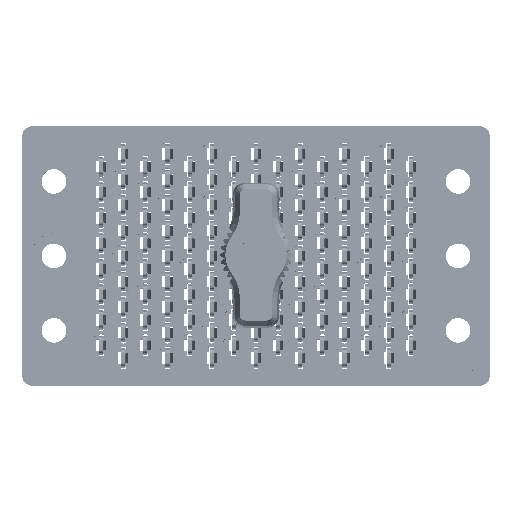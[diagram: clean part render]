
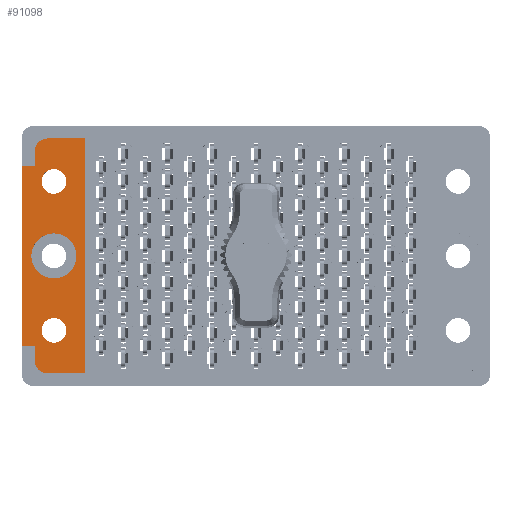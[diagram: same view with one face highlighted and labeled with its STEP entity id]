
A CAD part, top view. The second image highlights one B-rep face of the part: STEP entity #91098.
In plain terms, the highlighted planar face has unit normal (0, 0, 1).
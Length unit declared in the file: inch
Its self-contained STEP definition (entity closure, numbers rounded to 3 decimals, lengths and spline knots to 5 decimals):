
#520 = EDGE_CURVE ( 'NONE', #76508, #47796, #1951, .T. ) ;
#1688 = CARTESIAN_POINT ( 'NONE',  ( -1.3, 0.5285, -0.117 ) ) ;
#1951 = LINE ( 'NONE', #77015, #81030 ) ;
#3265 = VERTEX_POINT ( 'NONE', #38619 ) ;
#3399 = CARTESIAN_POINT ( 'NONE',  ( -1.225, -0.615, -0.117 ) ) ;
#4760 = VECTOR ( 'NONE', #86112, 39.37008 ) ;
#5587 = DIRECTION ( 'NONE',  ( 1., 0., 0. ) ) ;
#7339 = CARTESIAN_POINT ( 'NONE',  ( -1.3, -0.615, -0.117 ) ) ;
#7540 = DIRECTION ( 'NONE',  ( -1., 0., 0. ) ) ;
#8501 = VERTEX_POINT ( 'NONE', #13910 ) ;
#8773 = EDGE_LOOP ( 'NONE', ( #49621, #72339 ) ) ;
#10716 = DIRECTION ( 'NONE',  ( 0., 0., 1. ) ) ;
#10899 = VERTEX_POINT ( 'NONE', #83333 ) ;
#11388 = DIRECTION ( 'NONE',  ( -1., 0., 0. ) ) ;
#11591 = EDGE_LOOP ( 'NONE', ( #106230, #72135 ) ) ;
#11760 = CARTESIAN_POINT ( 'NONE',  ( 0., 0.69, -0.117 ) ) ;
#11812 = VERTEX_POINT ( 'NONE', #95992 ) ;
#11951 = AXIS2_PLACEMENT_3D ( 'NONE', #38416, #14511, #63714 ) ;
#12415 = VERTEX_POINT ( 'NONE', #104244 ) ;
#12873 = VECTOR ( 'NONE', #105240, 39.37008 ) ;
#13069 = VERTEX_POINT ( 'NONE', #104713 ) ;
#13159 = VERTEX_POINT ( 'NONE', #7339 ) ;
#13910 = CARTESIAN_POINT ( 'NONE',  ( -1.115, 0.4375, -0.117 ) ) ;
#14511 = DIRECTION ( 'NONE',  ( 0., 0., 1. ) ) ;
#15698 = EDGE_CURVE ( 'NONE', #92973, #13069, #87739, .T. ) ;
#16924 = ORIENTED_EDGE ( 'NONE', *, *, #95785, .F. ) ;
#18304 = CIRCLE ( 'NONE', #53966, 0.1325 ) ;
#19270 = DIRECTION ( 'NONE',  ( 1., 0., 0. ) ) ;
#19272 = VECTOR ( 'NONE', #11388, 39.37008 ) ;
#19824 = DIRECTION ( 'NONE',  ( 1., 0., 0. ) ) ;
#19916 = FACE_OUTER_BOUND ( 'NONE', #60039, .T. ) ;
#21503 = ORIENTED_EDGE ( 'NONE', *, *, #50253, .T. ) ;
#21797 = VECTOR ( 'NONE', #71695, 39.37008 ) ;
#23635 = VERTEX_POINT ( 'NONE', #99244 ) ;
#23939 = CARTESIAN_POINT ( 'NONE',  ( -1.1875, -0.4375, -0.117 ) ) ;
#25273 = CARTESIAN_POINT ( 'NONE',  ( -1.26, 0.4375, -0.117 ) ) ;
#25336 = CIRCLE ( 'NONE', #72928, 0.1325 ) ;
#26126 = ORIENTED_EDGE ( 'NONE', *, *, #47412, .T. ) ;
#26280 = EDGE_CURVE ( 'NONE', #12415, #13069, #29616, .T. ) ;
#27283 = DIRECTION ( 'NONE',  ( -1., 0., 0. ) ) ;
#29616 = LINE ( 'NONE', #39129, #21797 ) ;
#31149 = CARTESIAN_POINT ( 'NONE',  ( -1.3, 0., -0.117 ) ) ;
#32296 = LINE ( 'NONE', #31149, #12873 ) ;
#33438 = ORIENTED_EDGE ( 'NONE', *, *, #57508, .T. ) ;
#35520 = FACE_BOUND ( 'NONE', #8773, .T. ) ;
#35893 = CARTESIAN_POINT ( 'NONE',  ( -1.1875, 0.4375, -0.117 ) ) ;
#35933 = ORIENTED_EDGE ( 'NONE', *, *, #520, .T. ) ;
#36636 = EDGE_CURVE ( 'NONE', #92973, #13159, #32296, .T. ) ;
#38324 = VECTOR ( 'NONE', #40312, 39.37008 ) ;
#38416 = CARTESIAN_POINT ( 'NONE',  ( -1.225, 0.615, -0.117 ) ) ;
#38619 = CARTESIAN_POINT ( 'NONE',  ( -1.005, -0.69, -0.117 ) ) ;
#38698 = LINE ( 'NONE', #11760, #19272 ) ;
#39129 = CARTESIAN_POINT ( 'NONE',  ( -1.375, 0.7625, -0.117 ) ) ;
#39452 = CARTESIAN_POINT ( 'NONE',  ( -1.32, 0., -0.117 ) ) ;
#40312 = DIRECTION ( 'NONE',  ( -1., 0., 0. ) ) ;
#44028 = VERTEX_POINT ( 'NONE', #53080 ) ;
#44080 = CARTESIAN_POINT ( 'NONE',  ( -1.1875, 0.4375, -0.117 ) ) ;
#45246 = AXIS2_PLACEMENT_3D ( 'NONE', #35893, #102063, #95484 ) ;
#46981 = DIRECTION ( 'NONE',  ( 0., 0., 1. ) ) ;
#47282 = CIRCLE ( 'NONE', #86715, 0.0725 ) ;
#47412 = EDGE_CURVE ( 'NONE', #47796, #12415, #101451, .T. ) ;
#47796 = VERTEX_POINT ( 'NONE', #1688 ) ;
#48241 = ORIENTED_EDGE ( 'NONE', *, *, #80964, .T. ) ;
#48360 = CARTESIAN_POINT ( 'NONE',  ( -1.375, -0.7625, -0.117 ) ) ;
#49254 = CARTESIAN_POINT ( 'NONE',  ( 0., -0.5285, -0.117 ) ) ;
#49621 = ORIENTED_EDGE ( 'NONE', *, *, #85861, .F. ) ;
#50253 = EDGE_CURVE ( 'NONE', #13159, #10899, #79186, .T. ) ;
#50691 = CARTESIAN_POINT ( 'NONE',  ( -1.3, 0.615, -0.117 ) ) ;
#52391 = EDGE_CURVE ( 'NONE', #3265, #95756, #52895, .T. ) ;
#52895 = LINE ( 'NONE', #77806, #4760 ) ;
#53080 = CARTESIAN_POINT ( 'NONE',  ( -1.26, -0.4375, -0.117 ) ) ;
#53904 = EDGE_CURVE ( 'NONE', #94583, #23635, #25336, .T. ) ;
#53966 = AXIS2_PLACEMENT_3D ( 'NONE', #76450, #102097, #101011 ) ;
#54897 = ORIENTED_EDGE ( 'NONE', *, *, #26280, .T. ) ;
#56177 = FACE_BOUND ( 'NONE', #96705, .T. ) ;
#56354 = DIRECTION ( 'NONE',  ( 0., 0., 1. ) ) ;
#57066 = AXIS2_PLACEMENT_3D ( 'NONE', #48360, #56354, #5587 ) ;
#57508 = EDGE_CURVE ( 'NONE', #95756, #11812, #38698, .T. ) ;
#57691 = CIRCLE ( 'NONE', #11951, 0.075 ) ;
#58684 = EDGE_CURVE ( 'NONE', #90835, #8501, #61764, .T. ) ;
#60039 = EDGE_LOOP ( 'NONE', ( #33438, #48241, #35933, #26126, #54897, #75944, #79755, #21503, #16924, #84002 ) ) ;
#60347 = LINE ( 'NONE', #89783, #38324 ) ;
#60556 = DIRECTION ( 'NONE',  ( 0., 0., 1. ) ) ;
#60776 = AXIS2_PLACEMENT_3D ( 'NONE', #101778, #60556, #19270 ) ;
#61764 = CIRCLE ( 'NONE', #91225, 0.0725 ) ;
#63612 = DIRECTION ( 'NONE',  ( 1., 0., 0. ) ) ;
#63714 = DIRECTION ( 'NONE',  ( 1., 0., 0. ) ) ;
#65769 = VECTOR ( 'NONE', #7540, 39.37008 ) ;
#68951 = VECTOR ( 'NONE', #27283, 39.37008 ) ;
#69592 = ORIENTED_EDGE ( 'NONE', *, *, #80923, .F. ) ;
#71034 = DIRECTION ( 'NONE',  ( 0., -1., 0. ) ) ;
#71695 = DIRECTION ( 'NONE',  ( 0., -1., 0. ) ) ;
#71731 = CIRCLE ( 'NONE', #60776, 0.0725 ) ;
#71982 = AXIS2_PLACEMENT_3D ( 'NONE', #3399, #10716, #102224 ) ;
#72135 = ORIENTED_EDGE ( 'NONE', *, *, #53904, .F. ) ;
#72339 = ORIENTED_EDGE ( 'NONE', *, *, #80470, .F. ) ;
#72928 = AXIS2_PLACEMENT_3D ( 'NONE', #87815, #46981, #63612 ) ;
#75839 = CIRCLE ( 'NONE', #45246, 0.0725 ) ;
#75944 = ORIENTED_EDGE ( 'NONE', *, *, #15698, .F. ) ;
#76450 = CARTESIAN_POINT ( 'NONE',  ( -1.1875, 0., -0.117 ) ) ;
#76508 = VERTEX_POINT ( 'NONE', #50691 ) ;
#77015 = CARTESIAN_POINT ( 'NONE',  ( -1.3, 0., -0.117 ) ) ;
#77806 = CARTESIAN_POINT ( 'NONE',  ( -1.005, 0.7625, -0.117 ) ) ;
#79186 = CIRCLE ( 'NONE', #71982, 0.075 ) ;
#79755 = ORIENTED_EDGE ( 'NONE', *, *, #36636, .T. ) ;
#80113 = CARTESIAN_POINT ( 'NONE',  ( -1.005, 0.69, -0.117 ) ) ;
#80470 = EDGE_CURVE ( 'NONE', #88556, #44028, #47282, .T. ) ;
#80897 = PLANE ( 'NONE',  #57066 ) ;
#80923 = EDGE_CURVE ( 'NONE', #8501, #90835, #75839, .T. ) ;
#80964 = EDGE_CURVE ( 'NONE', #11812, #76508, #57691, .T. ) ;
#81030 = VECTOR ( 'NONE', #71034, 39.37008 ) ;
#82135 = DIRECTION ( 'NONE',  ( 0., 0., 1. ) ) ;
#83333 = CARTESIAN_POINT ( 'NONE',  ( -1.225, -0.69, -0.117 ) ) ;
#84002 = ORIENTED_EDGE ( 'NONE', *, *, #52391, .T. ) ;
#85861 = EDGE_CURVE ( 'NONE', #44028, #88556, #71731, .T. ) ;
#86112 = DIRECTION ( 'NONE',  ( 0., 1., 0. ) ) ;
#86715 = AXIS2_PLACEMENT_3D ( 'NONE', #23939, #82135, #89000 ) ;
#87248 = CARTESIAN_POINT ( 'NONE',  ( -1.115, -0.4375, -0.117 ) ) ;
#87575 = EDGE_CURVE ( 'NONE', #23635, #94583, #18304, .T. ) ;
#87739 = LINE ( 'NONE', #49254, #65769 ) ;
#87815 = CARTESIAN_POINT ( 'NONE',  ( -1.1875, 0., -0.117 ) ) ;
#88556 = VERTEX_POINT ( 'NONE', #87248 ) ;
#89000 = DIRECTION ( 'NONE',  ( 1., 0., 0. ) ) ;
#89783 = CARTESIAN_POINT ( 'NONE',  ( 0., -0.69, -0.117 ) ) ;
#90835 = VERTEX_POINT ( 'NONE', #25273 ) ;
#91098 = ADVANCED_FACE ( 'NONE', ( #56177, #35520, #96252, #19916 ), #80897, .T. ) ;
#91176 = ORIENTED_EDGE ( 'NONE', *, *, #58684, .F. ) ;
#91225 = AXIS2_PLACEMENT_3D ( 'NONE', #44080, #94287, #19824 ) ;
#92703 = CARTESIAN_POINT ( 'NONE',  ( -1.3, -0.5285, -0.117 ) ) ;
#92973 = VERTEX_POINT ( 'NONE', #92703 ) ;
#94287 = DIRECTION ( 'NONE',  ( 0., 0., 1. ) ) ;
#94583 = VERTEX_POINT ( 'NONE', #39452 ) ;
#95484 = DIRECTION ( 'NONE',  ( 1., 0., 0. ) ) ;
#95756 = VERTEX_POINT ( 'NONE', #80113 ) ;
#95785 = EDGE_CURVE ( 'NONE', #3265, #10899, #60347, .T. ) ;
#95992 = CARTESIAN_POINT ( 'NONE',  ( -1.225, 0.69, -0.117 ) ) ;
#96252 = FACE_BOUND ( 'NONE', #11591, .T. ) ;
#96705 = EDGE_LOOP ( 'NONE', ( #91176, #69592 ) ) ;
#99244 = CARTESIAN_POINT ( 'NONE',  ( -1.055, 0., -0.117 ) ) ;
#101011 = DIRECTION ( 'NONE',  ( 1., 0., 0. ) ) ;
#101044 = CARTESIAN_POINT ( 'NONE',  ( 0., 0.5285, -0.117 ) ) ;
#101451 = LINE ( 'NONE', #101044, #68951 ) ;
#101778 = CARTESIAN_POINT ( 'NONE',  ( -1.1875, -0.4375, -0.117 ) ) ;
#102063 = DIRECTION ( 'NONE',  ( 0., 0., 1. ) ) ;
#102097 = DIRECTION ( 'NONE',  ( 0., 0., 1. ) ) ;
#102224 = DIRECTION ( 'NONE',  ( 1., 0., 0. ) ) ;
#104244 = CARTESIAN_POINT ( 'NONE',  ( -1.375, 0.5285, -0.117 ) ) ;
#104713 = CARTESIAN_POINT ( 'NONE',  ( -1.375, -0.5285, -0.117 ) ) ;
#105240 = DIRECTION ( 'NONE',  ( 0., -1., 0. ) ) ;
#106230 = ORIENTED_EDGE ( 'NONE', *, *, #87575, .F. ) ;
